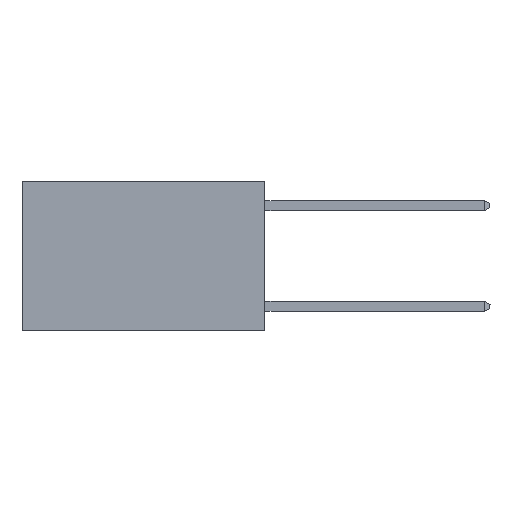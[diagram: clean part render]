
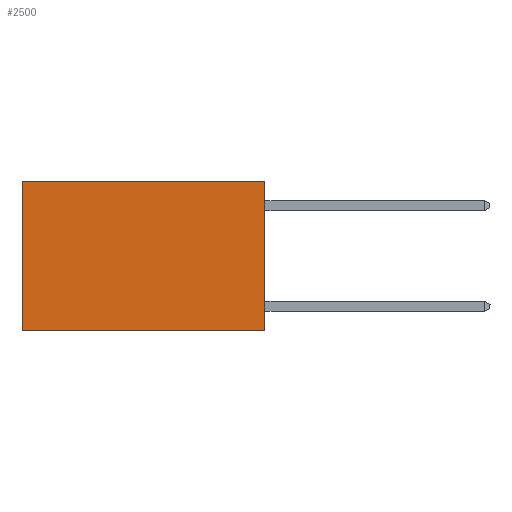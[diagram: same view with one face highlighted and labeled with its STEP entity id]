
A CAD part, left-side view. The second image highlights one B-rep face of the part: STEP entity #2500.
In plain terms, the highlighted planar face has unit normal (-1, 0, 0).
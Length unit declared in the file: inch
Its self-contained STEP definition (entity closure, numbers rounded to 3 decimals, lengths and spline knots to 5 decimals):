
#40 = AXIS2_PLACEMENT_3D ( 'NONE', #5285, #1370, #6077 ) ;
#179 = LINE ( 'NONE', #826, #7590 ) ;
#240 = DIRECTION ( 'NONE',  ( 0., 0., -1. ) ) ;
#304 = LINE ( 'NONE', #3804, #1863 ) ;
#382 = LINE ( 'NONE', #7243, #5387 ) ;
#454 = VERTEX_POINT ( 'NONE', #827 ) ;
#554 = EDGE_CURVE ( 'NONE', #454, #2888, #382, .T. ) ;
#826 = CARTESIAN_POINT ( 'NONE',  ( 0.2625, 0., -0.37 ) ) ;
#827 = CARTESIAN_POINT ( 'NONE',  ( 0.2625, 0., 0. ) ) ;
#902 = ORIENTED_EDGE ( 'NONE', *, *, #5124, .T. ) ;
#1370 = DIRECTION ( 'NONE',  ( 1., 0., 0. ) ) ;
#1516 = ORIENTED_EDGE ( 'NONE', *, *, #7586, .T. ) ;
#1599 = CARTESIAN_POINT ( 'NONE',  ( 0.2625, 0., -0.37 ) ) ;
#1863 = VECTOR ( 'NONE', #7544, 39.37008 ) ;
#2355 = LINE ( 'NONE', #6506, #9535 ) ;
#2376 = PLANE ( 'NONE',  #40 ) ;
#2500 = ADVANCED_FACE ( 'NONE', ( #3856 ), #2376, .F. ) ;
#2516 = DIRECTION ( 'NONE',  ( 0., 1., 0. ) ) ;
#2860 = VERTEX_POINT ( 'NONE', #4079 ) ;
#2888 = VERTEX_POINT ( 'NONE', #1599 ) ;
#3149 = EDGE_LOOP ( 'NONE', ( #1516, #9924, #7504, #902 ) ) ;
#3804 = CARTESIAN_POINT ( 'NONE',  ( 0.2625, 0.6, 0. ) ) ;
#3856 = FACE_OUTER_BOUND ( 'NONE', #3149, .T. ) ;
#4079 = CARTESIAN_POINT ( 'NONE',  ( 0.2625, 0.6, -0.37 ) ) ;
#4270 = DIRECTION ( 'NONE',  ( 0., 1., 0. ) ) ;
#5124 = EDGE_CURVE ( 'NONE', #454, #7192, #2355, .T. ) ;
#5285 = CARTESIAN_POINT ( 'NONE',  ( 0.2625, 0., 0. ) ) ;
#5387 = VECTOR ( 'NONE', #240, 39.37008 ) ;
#6077 = DIRECTION ( 'NONE',  ( 0., 0., -1. ) ) ;
#6431 = EDGE_CURVE ( 'NONE', #2888, #2860, #179, .T. ) ;
#6506 = CARTESIAN_POINT ( 'NONE',  ( 0.2625, 0., 0. ) ) ;
#7192 = VERTEX_POINT ( 'NONE', #7562 ) ;
#7243 = CARTESIAN_POINT ( 'NONE',  ( 0.2625, 0., 0. ) ) ;
#7504 = ORIENTED_EDGE ( 'NONE', *, *, #554, .F. ) ;
#7544 = DIRECTION ( 'NONE',  ( 0., 0., -1. ) ) ;
#7562 = CARTESIAN_POINT ( 'NONE',  ( 0.2625, 0.6, 0. ) ) ;
#7586 = EDGE_CURVE ( 'NONE', #7192, #2860, #304, .T. ) ;
#7590 = VECTOR ( 'NONE', #2516, 39.37008 ) ;
#9535 = VECTOR ( 'NONE', #4270, 39.37008 ) ;
#9924 = ORIENTED_EDGE ( 'NONE', *, *, #6431, .F. ) ;
